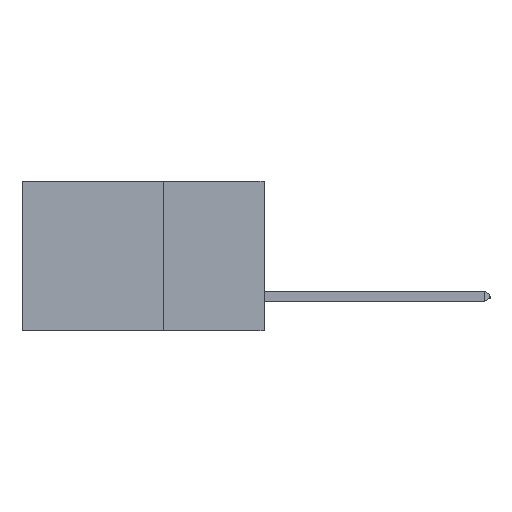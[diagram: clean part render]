
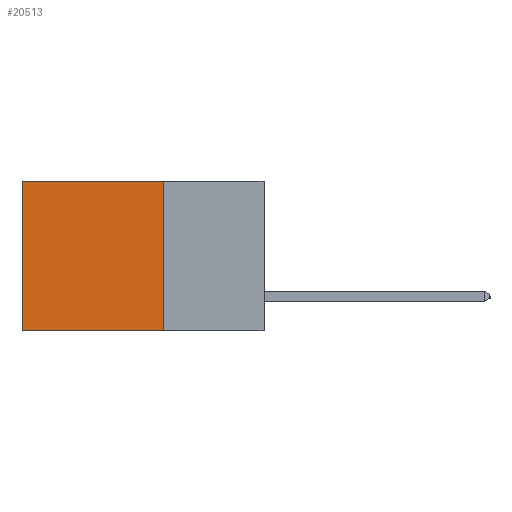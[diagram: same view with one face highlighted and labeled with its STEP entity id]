
A CAD part, left-side view. The second image highlights one B-rep face of the part: STEP entity #20513.
In plain terms, the highlighted planar face has unit normal (-1, 0, 0).
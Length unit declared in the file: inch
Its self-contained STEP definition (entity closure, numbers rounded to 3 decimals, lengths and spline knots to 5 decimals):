
#127 = CARTESIAN_POINT ( 'NONE',  ( 0.298, 0.25, 0. ) ) ;
#412 = CARTESIAN_POINT ( 'NONE',  ( 0.298, 0.25, 0. ) ) ;
#705 = CARTESIAN_POINT ( 'NONE',  ( 0.298, 0.6, 0. ) ) ;
#1068 = VECTOR ( 'NONE', #16992, 39.37008 ) ;
#1354 = VECTOR ( 'NONE', #20302, 39.37008 ) ;
#3376 = PLANE ( 'NONE',  #3478 ) ;
#3478 = AXIS2_PLACEMENT_3D ( 'NONE', #21338, #23066, #12556 ) ;
#4746 = EDGE_LOOP ( 'NONE', ( #18150, #17016, #9893, #9736 ) ) ;
#6241 = VECTOR ( 'NONE', #12105, 39.37008 ) ;
#6556 = VERTEX_POINT ( 'NONE', #12876 ) ;
#6664 = LINE ( 'NONE', #705, #1068 ) ;
#6930 = CARTESIAN_POINT ( 'NONE',  ( 0.298, 0.6, -0.37 ) ) ;
#7599 = DIRECTION ( 'NONE',  ( 0., 1., 0. ) ) ;
#7859 = CARTESIAN_POINT ( 'NONE',  ( 0.298, 0.6, 0. ) ) ;
#9288 = FACE_OUTER_BOUND ( 'NONE', #4746, .T. ) ;
#9736 = ORIENTED_EDGE ( 'NONE', *, *, #17999, .T. ) ;
#9764 = CARTESIAN_POINT ( 'NONE',  ( 0.298, 0.25, 0. ) ) ;
#9893 = ORIENTED_EDGE ( 'NONE', *, *, #21455, .F. ) ;
#10715 = VECTOR ( 'NONE', #7599, 39.37008 ) ;
#11701 = EDGE_CURVE ( 'NONE', #6556, #16796, #15698, .T. ) ;
#11753 = LINE ( 'NONE', #9764, #1354 ) ;
#12105 = DIRECTION ( 'NONE',  ( 0., 1., 0. ) ) ;
#12556 = DIRECTION ( 'NONE',  ( 0., 0., -1. ) ) ;
#12876 = CARTESIAN_POINT ( 'NONE',  ( 0.298, 0.25, -0.37 ) ) ;
#15698 = LINE ( 'NONE', #19092, #6241 ) ;
#15909 = LINE ( 'NONE', #127, #10715 ) ;
#16796 = VERTEX_POINT ( 'NONE', #6930 ) ;
#16992 = DIRECTION ( 'NONE',  ( 0., 0., -1. ) ) ;
#17016 = ORIENTED_EDGE ( 'NONE', *, *, #11701, .F. ) ;
#17452 = VERTEX_POINT ( 'NONE', #7859 ) ;
#17999 = EDGE_CURVE ( 'NONE', #20728, #17452, #15909, .T. ) ;
#18150 = ORIENTED_EDGE ( 'NONE', *, *, #19344, .T. ) ;
#19092 = CARTESIAN_POINT ( 'NONE',  ( 0.298, 0.25, -0.37 ) ) ;
#19344 = EDGE_CURVE ( 'NONE', #17452, #16796, #6664, .T. ) ;
#20302 = DIRECTION ( 'NONE',  ( 0., 0., -1. ) ) ;
#20513 = ADVANCED_FACE ( 'NONE', ( #9288 ), #3376, .F. ) ;
#20728 = VERTEX_POINT ( 'NONE', #412 ) ;
#21338 = CARTESIAN_POINT ( 'NONE',  ( 0.298, 0.25, 0. ) ) ;
#21455 = EDGE_CURVE ( 'NONE', #20728, #6556, #11753, .T. ) ;
#23066 = DIRECTION ( 'NONE',  ( 1., 0., 0. ) ) ;
